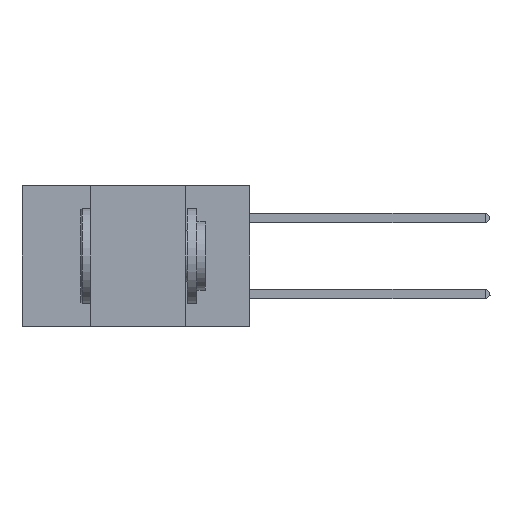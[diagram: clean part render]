
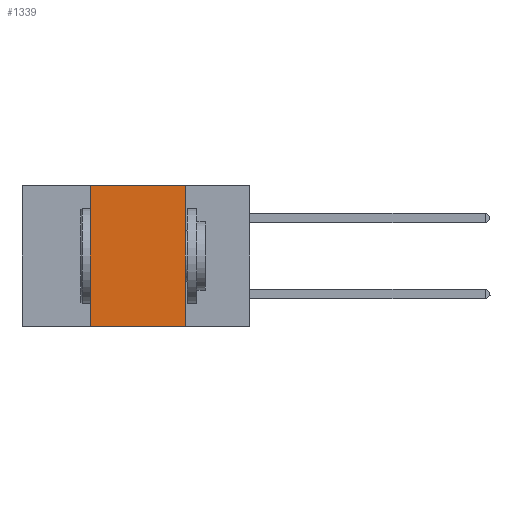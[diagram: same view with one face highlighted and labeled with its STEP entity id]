
A CAD part, left-side view. The second image highlights one B-rep face of the part: STEP entity #1339.
In plain terms, the highlighted planar face has unit normal (-1, 0, 0).
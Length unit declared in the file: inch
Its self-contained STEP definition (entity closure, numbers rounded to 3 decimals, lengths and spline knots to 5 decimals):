
#956 = EDGE_CURVE ( 'NONE', #17945, #25793, #18780, .T. ) ;
#1339 = ADVANCED_FACE ( 'NONE', ( #23810 ), #12734, .F. ) ;
#4377 = VECTOR ( 'NONE', #35114, 39.37008 ) ;
#11421 = ORIENTED_EDGE ( 'NONE', *, *, #36282, .T. ) ;
#12734 = PLANE ( 'NONE',  #15250 ) ;
#12967 = LINE ( 'NONE', #21497, #34579 ) ;
#14738 = VECTOR ( 'NONE', #16932, 39.37008 ) ;
#14766 = EDGE_CURVE ( 'NONE', #32055, #37431, #12967, .T. ) ;
#15250 = AXIS2_PLACEMENT_3D ( 'NONE', #28640, #31458, #24967 ) ;
#16932 = DIRECTION ( 'NONE',  ( 0., 0., -1. ) ) ;
#17945 = VERTEX_POINT ( 'NONE', #33128 ) ;
#17980 = DIRECTION ( 'NONE',  ( 0., 0., 1. ) ) ;
#18575 = ORIENTED_EDGE ( 'NONE', *, *, #14766, .F. ) ;
#18780 = LINE ( 'NONE', #36227, #14738 ) ;
#21431 = LINE ( 'NONE', #41318, #4377 ) ;
#21497 = CARTESIAN_POINT ( 'NONE',  ( 0., 0.42, 0. ) ) ;
#23120 = EDGE_LOOP ( 'NONE', ( #36029, #38527, #18575, #11421 ) ) ;
#23810 = FACE_OUTER_BOUND ( 'NONE', #23120, .T. ) ;
#24967 = DIRECTION ( 'NONE',  ( 0., 0., -1. ) ) ;
#25793 = VERTEX_POINT ( 'NONE', #36580 ) ;
#28640 = CARTESIAN_POINT ( 'NONE',  ( 0., 0.6, 0. ) ) ;
#29298 = DIRECTION ( 'NONE',  ( 0., -1., 0. ) ) ;
#30562 = CARTESIAN_POINT ( 'NONE',  ( 0., 0.42, 0. ) ) ;
#31278 = EDGE_CURVE ( 'NONE', #37431, #17945, #21431, .T. ) ;
#31458 = DIRECTION ( 'NONE',  ( 1., 0., 0. ) ) ;
#32055 = VERTEX_POINT ( 'NONE', #32975 ) ;
#32403 = CARTESIAN_POINT ( 'NONE',  ( 0., 0.6, -0.37 ) ) ;
#32975 = CARTESIAN_POINT ( 'NONE',  ( 0., 0.42, -0.37 ) ) ;
#33128 = CARTESIAN_POINT ( 'NONE',  ( 0., 0.17, 0. ) ) ;
#33820 = VECTOR ( 'NONE', #29298, 39.37008 ) ;
#34579 = VECTOR ( 'NONE', #17980, 39.37008 ) ;
#35114 = DIRECTION ( 'NONE',  ( 0., -1., 0. ) ) ;
#36029 = ORIENTED_EDGE ( 'NONE', *, *, #956, .F. ) ;
#36227 = CARTESIAN_POINT ( 'NONE',  ( 0., 0.17, 0. ) ) ;
#36282 = EDGE_CURVE ( 'NONE', #32055, #25793, #38892, .T. ) ;
#36580 = CARTESIAN_POINT ( 'NONE',  ( 0., 0.17, -0.37 ) ) ;
#37431 = VERTEX_POINT ( 'NONE', #30562 ) ;
#38527 = ORIENTED_EDGE ( 'NONE', *, *, #31278, .F. ) ;
#38892 = LINE ( 'NONE', #32403, #33820 ) ;
#41318 = CARTESIAN_POINT ( 'NONE',  ( 0., 0.6, 0. ) ) ;
